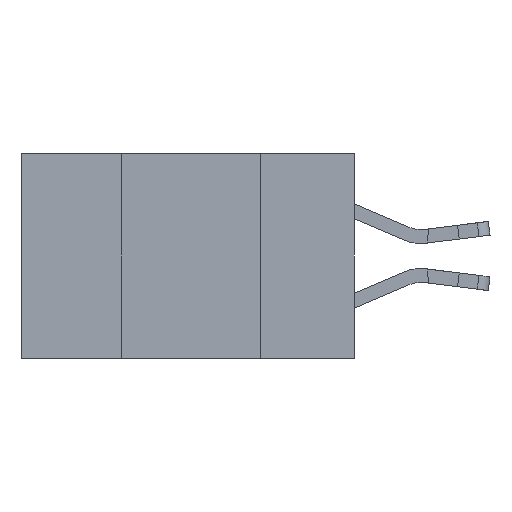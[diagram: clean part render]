
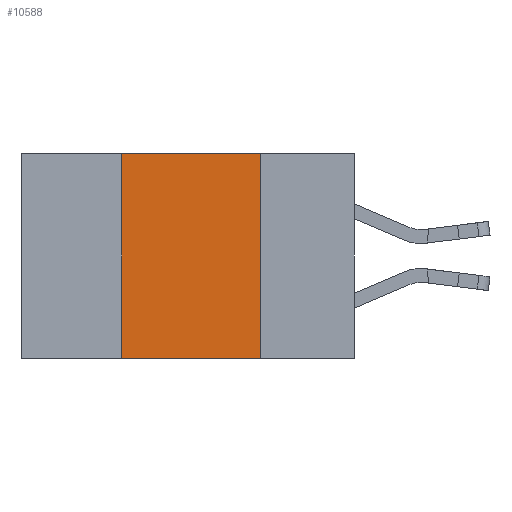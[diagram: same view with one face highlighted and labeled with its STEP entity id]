
A CAD part, left-side view. The second image highlights one B-rep face of the part: STEP entity #10588.
In plain terms, the highlighted planar face has unit normal (-1, 0, 0).
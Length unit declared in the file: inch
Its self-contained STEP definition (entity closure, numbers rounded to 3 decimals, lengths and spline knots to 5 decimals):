
#518 = CARTESIAN_POINT ( 'NONE',  ( 0., 0.42, -0.37 ) ) ;
#1278 = AXIS2_PLACEMENT_3D ( 'NONE', #6464, #5659, #11573 ) ;
#1392 = FACE_OUTER_BOUND ( 'NONE', #5814, .T. ) ;
#1523 = VERTEX_POINT ( 'NONE', #11147 ) ;
#1537 = PLANE ( 'NONE',  #1278 ) ;
#1698 = ORIENTED_EDGE ( 'NONE', *, *, #11105, .T. ) ;
#1716 = VECTOR ( 'NONE', #7879, 39.37008 ) ;
#1780 = ORIENTED_EDGE ( 'NONE', *, *, #12737, .F. ) ;
#3223 = LINE ( 'NONE', #9408, #11610 ) ;
#3642 = LINE ( 'NONE', #518, #5561 ) ;
#4172 = LINE ( 'NONE', #12534, #12982 ) ;
#4355 = DIRECTION ( 'NONE',  ( 0., 0., -1. ) ) ;
#5561 = VECTOR ( 'NONE', #7628, 39.37008 ) ;
#5659 = DIRECTION ( 'NONE',  ( 1., 0., 0. ) ) ;
#5814 = EDGE_LOOP ( 'NONE', ( #11549, #1780, #7142, #1698 ) ) ;
#6146 = CARTESIAN_POINT ( 'NONE',  ( 0., 0.17, -0.37 ) ) ;
#6316 = VERTEX_POINT ( 'NONE', #6146 ) ;
#6338 = EDGE_CURVE ( 'NONE', #7525, #6316, #3223, .T. ) ;
#6464 = CARTESIAN_POINT ( 'NONE',  ( 0., 0.6, 0. ) ) ;
#7142 = ORIENTED_EDGE ( 'NONE', *, *, #12334, .F. ) ;
#7525 = VERTEX_POINT ( 'NONE', #9832 ) ;
#7628 = DIRECTION ( 'NONE',  ( 0., 0., 1. ) ) ;
#7879 = DIRECTION ( 'NONE',  ( 0., -1., 0. ) ) ;
#8811 = LINE ( 'NONE', #13111, #1716 ) ;
#9408 = CARTESIAN_POINT ( 'NONE',  ( 0., 0.17, -0.37 ) ) ;
#9832 = CARTESIAN_POINT ( 'NONE',  ( 0., 0.17, 0. ) ) ;
#10461 = VERTEX_POINT ( 'NONE', #11251 ) ;
#10588 = ADVANCED_FACE ( 'NONE', ( #1392 ), #1537, .F. ) ;
#11105 = EDGE_CURVE ( 'NONE', #1523, #6316, #8811, .T. ) ;
#11147 = CARTESIAN_POINT ( 'NONE',  ( 0., 0.42, -0.37 ) ) ;
#11251 = CARTESIAN_POINT ( 'NONE',  ( 0., 0.42, 0. ) ) ;
#11549 = ORIENTED_EDGE ( 'NONE', *, *, #6338, .F. ) ;
#11573 = DIRECTION ( 'NONE',  ( 0., 0., -1. ) ) ;
#11610 = VECTOR ( 'NONE', #4355, 39.37008 ) ;
#12334 = EDGE_CURVE ( 'NONE', #1523, #10461, #3642, .T. ) ;
#12534 = CARTESIAN_POINT ( 'NONE',  ( 0., 0.6, 0. ) ) ;
#12737 = EDGE_CURVE ( 'NONE', #10461, #7525, #4172, .T. ) ;
#12900 = DIRECTION ( 'NONE',  ( 0., -1., 0. ) ) ;
#12982 = VECTOR ( 'NONE', #12900, 39.37008 ) ;
#13111 = CARTESIAN_POINT ( 'NONE',  ( 0., 0.6, -0.37 ) ) ;
